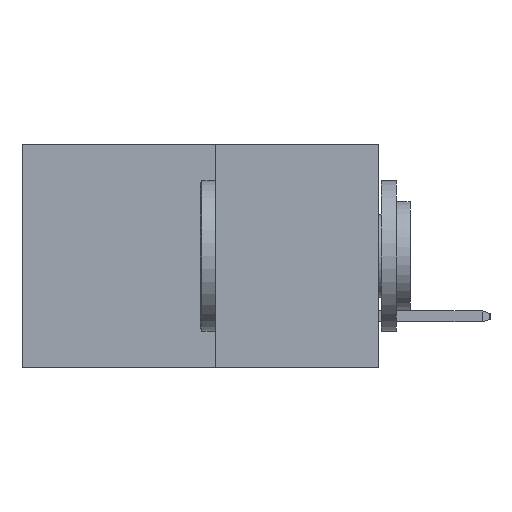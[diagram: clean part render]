
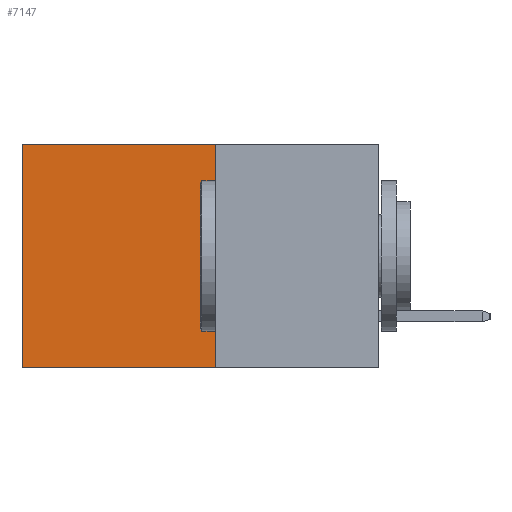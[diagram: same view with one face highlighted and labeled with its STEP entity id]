
A CAD part, left-side view. The second image highlights one B-rep face of the part: STEP entity #7147.
In plain terms, the highlighted planar face has unit normal (-1, 0, 0).
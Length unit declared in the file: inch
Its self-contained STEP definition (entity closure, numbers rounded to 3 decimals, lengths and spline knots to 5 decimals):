
#818 = VERTEX_POINT ( 'NONE', #4133 ) ;
#1151 = DIRECTION ( 'NONE',  ( 1., 0., 0. ) ) ;
#1306 = VECTOR ( 'NONE', #2521, 39.37008 ) ;
#1346 = CARTESIAN_POINT ( 'NONE',  ( 0.277, 0.59, -0.37 ) ) ;
#1359 = FACE_OUTER_BOUND ( 'NONE', #8130, .T. ) ;
#1573 = LINE ( 'NONE', #1613, #1306 ) ;
#1602 = ORIENTED_EDGE ( 'NONE', *, *, #3447, .T. ) ;
#1613 = CARTESIAN_POINT ( 'NONE',  ( 0.277, 0.27, -0.37 ) ) ;
#1618 = CARTESIAN_POINT ( 'NONE',  ( 0.277, 0.59, -0.37 ) ) ;
#1653 = ORIENTED_EDGE ( 'NONE', *, *, #9340, .F. ) ;
#1695 = VERTEX_POINT ( 'NONE', #6412 ) ;
#1705 = ORIENTED_EDGE ( 'NONE', *, *, #7927, .F. ) ;
#1726 = ORIENTED_EDGE ( 'NONE', *, *, #8885, .T. ) ;
#2158 = VERTEX_POINT ( 'NONE', #3366 ) ;
#2521 = DIRECTION ( 'NONE',  ( 0., 1., 0. ) ) ;
#3366 = CARTESIAN_POINT ( 'NONE',  ( 0.277, 0.27, 0. ) ) ;
#3447 = EDGE_CURVE ( 'NONE', #818, #8620, #6316, .T. ) ;
#3818 = VECTOR ( 'NONE', #9840, 39.37008 ) ;
#3822 = DIRECTION ( 'NONE',  ( 0., 0., -1. ) ) ;
#4133 = CARTESIAN_POINT ( 'NONE',  ( 0.277, 0.59, 0. ) ) ;
#4952 = AXIS2_PLACEMENT_3D ( 'NONE', #6032, #1151, #6825 ) ;
#5192 = CARTESIAN_POINT ( 'NONE',  ( 0.277, 0.27, 0. ) ) ;
#5830 = VECTOR ( 'NONE', #6999, 39.37008 ) ;
#6032 = CARTESIAN_POINT ( 'NONE',  ( 0.277, 0.27, -0.37 ) ) ;
#6316 = LINE ( 'NONE', #1618, #5830 ) ;
#6412 = CARTESIAN_POINT ( 'NONE',  ( 0.277, 0.27, -0.37 ) ) ;
#6825 = DIRECTION ( 'NONE',  ( 0., 0., -1. ) ) ;
#6912 = LINE ( 'NONE', #10018, #8975 ) ;
#6999 = DIRECTION ( 'NONE',  ( 0., 0., -1. ) ) ;
#7147 = ADVANCED_FACE ( 'NONE', ( #1359 ), #9132, .F. ) ;
#7927 = EDGE_CURVE ( 'NONE', #2158, #1695, #6912, .T. ) ;
#8002 = LINE ( 'NONE', #5192, #3818 ) ;
#8130 = EDGE_LOOP ( 'NONE', ( #1602, #1653, #1705, #1726 ) ) ;
#8620 = VERTEX_POINT ( 'NONE', #1346 ) ;
#8885 = EDGE_CURVE ( 'NONE', #2158, #818, #8002, .T. ) ;
#8975 = VECTOR ( 'NONE', #3822, 39.37008 ) ;
#9132 = PLANE ( 'NONE',  #4952 ) ;
#9340 = EDGE_CURVE ( 'NONE', #1695, #8620, #1573, .T. ) ;
#9840 = DIRECTION ( 'NONE',  ( 0., 1., 0. ) ) ;
#10018 = CARTESIAN_POINT ( 'NONE',  ( 0.277, 0.27, -0.37 ) ) ;
